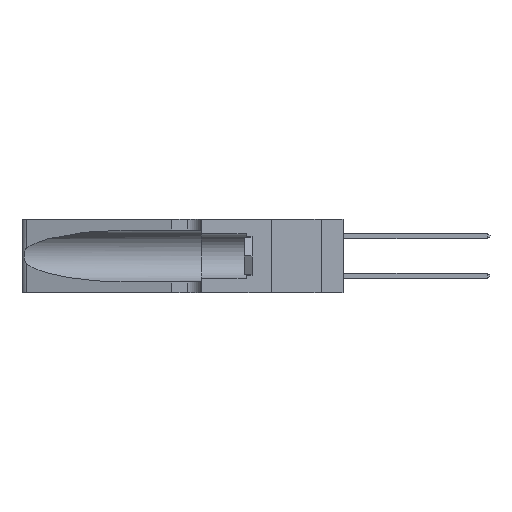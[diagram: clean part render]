
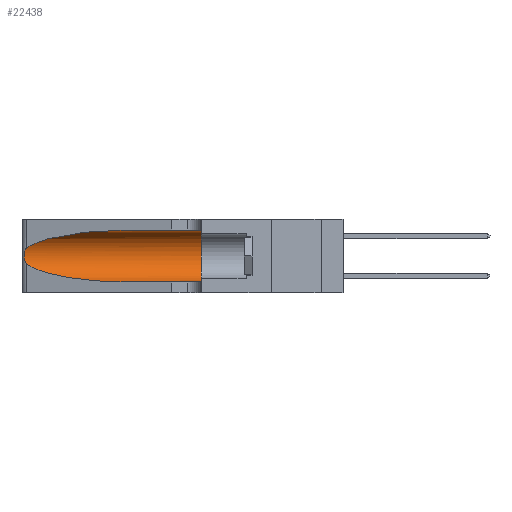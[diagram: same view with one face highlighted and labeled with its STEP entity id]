
A CAD part, left-side view. The second image highlights one B-rep face of the part: STEP entity #22438.
In plain terms, the highlighted cylindrical face has radius 3.308 mm (diameter 6.617 mm), a partial arc.
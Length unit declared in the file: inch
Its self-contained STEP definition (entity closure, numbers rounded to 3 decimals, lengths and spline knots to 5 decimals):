
#972 = CARTESIAN_POINT ( 'NONE',  ( 0.25487, 1.22718, 0.14631 ) ) ;
#1630 = CARTESIAN_POINT ( 'NONE',  ( 0.1305, 0.72297, 0.05475 ) ) ;
#2314 = CARTESIAN_POINT ( 'NONE',  ( 0.25487, 1.22718, 0.22369 ) ) ;
#2457 = CARTESIAN_POINT ( 'NONE',  ( 0.25854, 1.2359, 0.20912 ) ) ;
#3338 = CARTESIAN_POINT ( 'NONE',  ( 0.25487, 1.22718, 0.14631 ) ) ;
#3542 = DIRECTION ( 'NONE',  ( 0., 1., 0. ) ) ;
#3749 = CARTESIAN_POINT ( 'NONE',  ( 0.18966, 0.96281, 0.05475 ) ) ;
#3821 = LINE ( 'NONE', #37858, #5212 ) ;
#5212 = VECTOR ( 'NONE', #13463, 39.37008 ) ;
#5270 = CYLINDRICAL_SURFACE ( 'NONE', #8785, 0.13025 ) ;
#5336 = CARTESIAN_POINT ( 'NONE',  ( 0.18966, 0.96281, 0.31525 ) ) ;
#5484 = CARTESIAN_POINT ( 'NONE',  ( 0.26075, 1.23896, 0.19203 ) ) ;
#6620 = AXIS2_PLACEMENT_3D ( 'NONE', #36964, #3542, #10018 ) ;
#7081 =( BOUNDED_CURVE ( )  B_SPLINE_CURVE ( 3, ( #972, #34131, #3749, #1630 ),
 .UNSPECIFIED., .F., .T. ) 
 B_SPLINE_CURVE_WITH_KNOTS ( ( 4, 4 ),
 ( 3.44316, 4.71239 ),
 .UNSPECIFIED. ) 
 CURVE ( )  GEOMETRIC_REPRESENTATION_ITEM ( )  RATIONAL_B_SPLINE_CURVE ( ( 1., 0.87, 0.87, 1. ) ) 
 REPRESENTATION_ITEM ( '' )  );
#7408 = VERTEX_POINT ( 'NONE', #3338 ) ;
#7615 = ORIENTED_EDGE ( 'NONE', *, *, #28293, .T. ) ;
#7815 = ORIENTED_EDGE ( 'NONE', *, *, #18894, .T. ) ;
#8023 = CIRCLE ( 'NONE', #6620, 0.13025 ) ;
#8739 = ORIENTED_EDGE ( 'NONE', *, *, #36986, .F. ) ;
#8785 = AXIS2_PLACEMENT_3D ( 'NONE', #17368, #35911, #11472 ) ;
#10018 = DIRECTION ( 'NONE',  ( 0., 0., 1. ) ) ;
#11093 = EDGE_CURVE ( 'NONE', #28831, #30289, #3821, .T. ) ;
#11387 = CARTESIAN_POINT ( 'NONE',  ( 0.2373, 1.15595, 0.28018 ) ) ;
#11472 = DIRECTION ( 'NONE',  ( 0., 0., -1. ) ) ;
#11504 = VERTEX_POINT ( 'NONE', #2314 ) ;
#12976 = VERTEX_POINT ( 'NONE', #31929 ) ;
#13463 = DIRECTION ( 'NONE',  ( 0., -1., 0. ) ) ;
#14124 = CARTESIAN_POINT ( 'NONE',  ( 0.1305, 0.72297, 0.31525 ) ) ;
#14451 = CARTESIAN_POINT ( 'NONE',  ( 0.1305, 0.72297, 0.05475 ) ) ;
#14679 = CARTESIAN_POINT ( 'NONE',  ( 0.25555, 1.22993, 0.14849 ) ) ;
#17368 = CARTESIAN_POINT ( 'NONE',  ( 0.1305, 1.61858, 0.185 ) ) ;
#17488 = FACE_OUTER_BOUND ( 'NONE', #29308, .T. ) ;
#17839 = CARTESIAN_POINT ( 'NONE',  ( 0.25639, 1.23184, 0.21858 ) ) ;
#18894 = EDGE_CURVE ( 'NONE', #7408, #28831, #7081, .T. ) ;
#20485 = CARTESIAN_POINT ( 'NONE',  ( 0.25487, 1.22718, 0.22369 ) ) ;
#20760 = CARTESIAN_POINT ( 'NONE',  ( 0.25787, 1.23484, 0.2124 ) ) ;
#22264 = B_SPLINE_CURVE_WITH_KNOTS ( 'NONE', 3,
 ( #20485, #32293, #17839, #20760, #2457, #38643, #5484, #32685, #23497, #38361, #23236, #32815, #14679, #35711 ),
 .UNSPECIFIED., .F., .F.,
 ( 4, 2, 2, 2, 2, 2, 4 ),
 ( 0., 0.00027, 0.00053, 0.00107, 0.0016, 0.00187, 0.00214 ),
 .UNSPECIFIED. ) ;
#22438 = ADVANCED_FACE ( 'NONE', ( #17488 ), #5270, .F. ) ;
#22808 = VECTOR ( 'NONE', #36052, 39.37008 ) ;
#23236 = CARTESIAN_POINT ( 'NONE',  ( 0.25789, 1.23486, 0.15765 ) ) ;
#23497 = CARTESIAN_POINT ( 'NONE',  ( 0.26017, 1.23833, 0.17102 ) ) ;
#25449 = CARTESIAN_POINT ( 'NONE',  ( 0.1305, 0.35, 0.31525 ) ) ;
#27859 = CARTESIAN_POINT ( 'NONE',  ( 0.1305, 0.35, 0.05475 ) ) ;
#28293 = EDGE_CURVE ( 'NONE', #11504, #7408, #22264, .T. ) ;
#28831 = VERTEX_POINT ( 'NONE', #14451 ) ;
#29308 = EDGE_LOOP ( 'NONE', ( #37418, #7615, #7815, #31983, #8739, #32188 ) ) ;
#29535 = EDGE_CURVE ( 'NONE', #12976, #37832, #34584, .T. ) ;
#30289 = VERTEX_POINT ( 'NONE', #27859 ) ;
#31929 = CARTESIAN_POINT ( 'NONE',  ( 0.1305, 0.72297, 0.31525 ) ) ;
#31983 = ORIENTED_EDGE ( 'NONE', *, *, #11093, .T. ) ;
#32120 =( BOUNDED_CURVE ( )  B_SPLINE_CURVE ( 3, ( #14124, #5336, #11387, #38611 ),
 .UNSPECIFIED., .F., .F. ) 
 B_SPLINE_CURVE_WITH_KNOTS ( ( 4, 4 ),
 ( 1.5708, 2.84003 ),
 .UNSPECIFIED. ) 
 CURVE ( )  GEOMETRIC_REPRESENTATION_ITEM ( )  RATIONAL_B_SPLINE_CURVE ( ( 1., 0.87, 0.87, 1. ) ) 
 REPRESENTATION_ITEM ( '' )  );
#32188 = ORIENTED_EDGE ( 'NONE', *, *, #29535, .F. ) ;
#32293 = CARTESIAN_POINT ( 'NONE',  ( 0.25555, 1.22994, 0.2215 ) ) ;
#32685 = CARTESIAN_POINT ( 'NONE',  ( 0.26075, 1.23896, 0.178 ) ) ;
#32815 = CARTESIAN_POINT ( 'NONE',  ( 0.25639, 1.23186, 0.15144 ) ) ;
#34131 = CARTESIAN_POINT ( 'NONE',  ( 0.2373, 1.15595, 0.08982 ) ) ;
#34584 = LINE ( 'NONE', #35932, #22808 ) ;
#35711 = CARTESIAN_POINT ( 'NONE',  ( 0.25487, 1.22718, 0.14631 ) ) ;
#35911 = DIRECTION ( 'NONE',  ( 0., -1., 0. ) ) ;
#35932 = CARTESIAN_POINT ( 'NONE',  ( 0.1305, 1.61858, 0.31525 ) ) ;
#36052 = DIRECTION ( 'NONE',  ( 0., -1., 0. ) ) ;
#36964 = CARTESIAN_POINT ( 'NONE',  ( 0.1305, 0.35, 0.185 ) ) ;
#36986 = EDGE_CURVE ( 'NONE', #37832, #30289, #8023, .T. ) ;
#37418 = ORIENTED_EDGE ( 'NONE', *, *, #38683, .T. ) ;
#37832 = VERTEX_POINT ( 'NONE', #25449 ) ;
#37858 = CARTESIAN_POINT ( 'NONE',  ( 0.1305, 1.61858, 0.05475 ) ) ;
#38361 = CARTESIAN_POINT ( 'NONE',  ( 0.25856, 1.23593, 0.16098 ) ) ;
#38611 = CARTESIAN_POINT ( 'NONE',  ( 0.25487, 1.22718, 0.22369 ) ) ;
#38643 = CARTESIAN_POINT ( 'NONE',  ( 0.26018, 1.23835, 0.19895 ) ) ;
#38683 = EDGE_CURVE ( 'NONE', #12976, #11504, #32120, .T. ) ;
